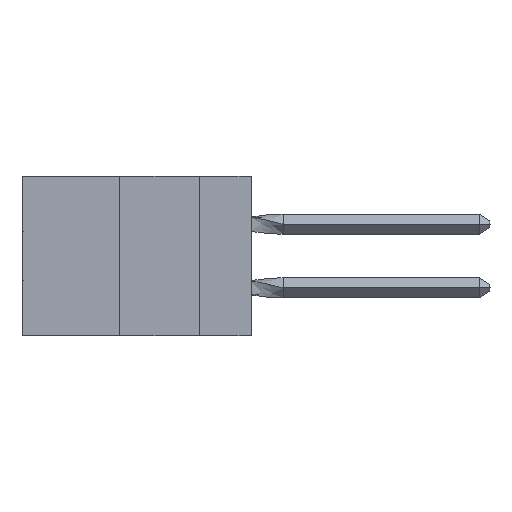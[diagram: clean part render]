
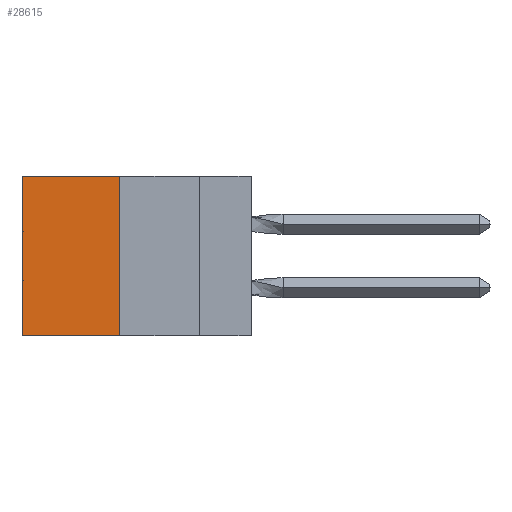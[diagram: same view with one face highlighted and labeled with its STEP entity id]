
A CAD part, left-side view. The second image highlights one B-rep face of the part: STEP entity #28615.
In plain terms, the highlighted planar face has unit normal (-1, 0, 0).
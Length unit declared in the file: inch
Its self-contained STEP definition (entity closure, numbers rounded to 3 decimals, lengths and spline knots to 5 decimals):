
#3394 = CARTESIAN_POINT ( 'NONE',  ( 0.305, 0.413, 0. ) ) ;
#4016 = CARTESIAN_POINT ( 'NONE',  ( 0.305, 0.413, -0.5 ) ) ;
#4104 = LINE ( 'NONE', #31385, #18633 ) ;
#7814 = CARTESIAN_POINT ( 'NONE',  ( 0.305, 0.413, -0.5 ) ) ;
#8409 = FACE_OUTER_BOUND ( 'NONE', #27500, .T. ) ;
#9716 = ORIENTED_EDGE ( 'NONE', *, *, #37226, .T. ) ;
#12488 = LINE ( 'NONE', #7814, #21252 ) ;
#16536 = VERTEX_POINT ( 'NONE', #22058 ) ;
#17499 = LINE ( 'NONE', #33937, #30872 ) ;
#17886 = CARTESIAN_POINT ( 'NONE',  ( 0.305, 0.413, 0. ) ) ;
#18012 = DIRECTION ( 'NONE',  ( 0., 0., -1. ) ) ;
#18066 = DIRECTION ( 'NONE',  ( 0., 1., 0. ) ) ;
#18332 = CARTESIAN_POINT ( 'NONE',  ( 0.305, 0.72, -0.5 ) ) ;
#18633 = VECTOR ( 'NONE', #18012, 39.37008 ) ;
#21252 = VECTOR ( 'NONE', #18066, 39.37008 ) ;
#22058 = CARTESIAN_POINT ( 'NONE',  ( 0.305, 0.413, -0.5 ) ) ;
#22318 = AXIS2_PLACEMENT_3D ( 'NONE', #4016, #33453, #36773 ) ;
#23001 = EDGE_CURVE ( 'NONE', #32024, #25050, #25902, .T. ) ;
#24872 = CARTESIAN_POINT ( 'NONE',  ( 0.305, 0.72, 0. ) ) ;
#25050 = VERTEX_POINT ( 'NONE', #24872 ) ;
#25902 = LINE ( 'NONE', #17886, #33188 ) ;
#27500 = EDGE_LOOP ( 'NONE', ( #9716, #38003, #34895, #38295 ) ) ;
#28615 = ADVANCED_FACE ( 'NONE', ( #8409 ), #33731, .F. ) ;
#28744 = EDGE_CURVE ( 'NONE', #16536, #32341, #12488, .T. ) ;
#29746 = EDGE_CURVE ( 'NONE', #32024, #16536, #4104, .T. ) ;
#30872 = VECTOR ( 'NONE', #34510, 39.37008 ) ;
#31385 = CARTESIAN_POINT ( 'NONE',  ( 0.305, 0.413, -0.5 ) ) ;
#32024 = VERTEX_POINT ( 'NONE', #3394 ) ;
#32341 = VERTEX_POINT ( 'NONE', #18332 ) ;
#33188 = VECTOR ( 'NONE', #37767, 39.37008 ) ;
#33453 = DIRECTION ( 'NONE',  ( 1., 0., 0. ) ) ;
#33731 = PLANE ( 'NONE',  #22318 ) ;
#33937 = CARTESIAN_POINT ( 'NONE',  ( 0.305, 0.72, -0.5 ) ) ;
#34510 = DIRECTION ( 'NONE',  ( 0., 0., -1. ) ) ;
#34895 = ORIENTED_EDGE ( 'NONE', *, *, #29746, .F. ) ;
#36773 = DIRECTION ( 'NONE',  ( 0., 0., -1. ) ) ;
#37226 = EDGE_CURVE ( 'NONE', #25050, #32341, #17499, .T. ) ;
#37767 = DIRECTION ( 'NONE',  ( 0., 1., 0. ) ) ;
#38003 = ORIENTED_EDGE ( 'NONE', *, *, #28744, .F. ) ;
#38295 = ORIENTED_EDGE ( 'NONE', *, *, #23001, .T. ) ;
